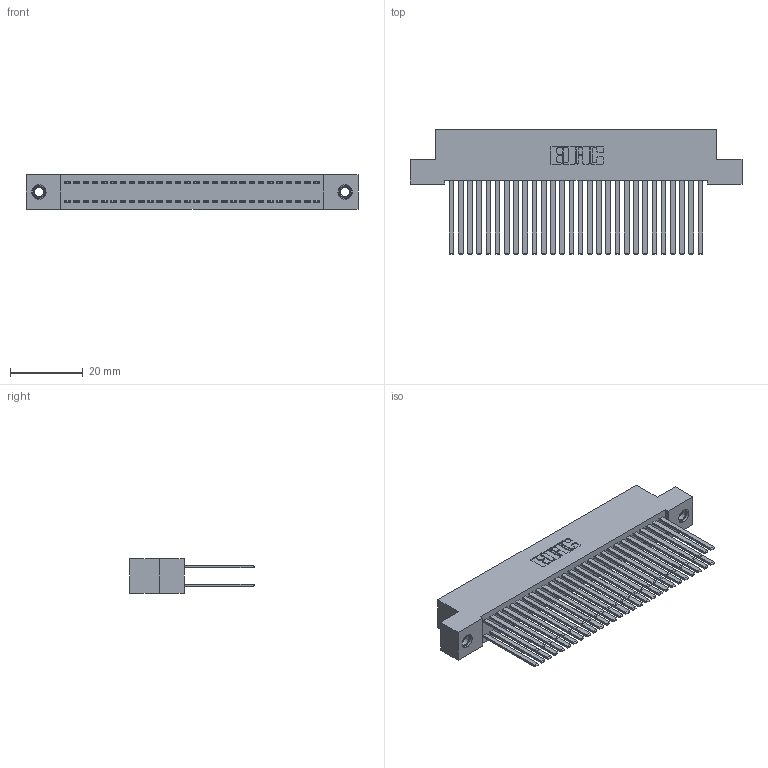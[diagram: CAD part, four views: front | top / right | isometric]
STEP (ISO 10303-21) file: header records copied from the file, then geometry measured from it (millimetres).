
FILE_DESCRIPTION (( 'STEP AP203' ), '1' );
FILE_NAME ('392-056-544-207.STEP', '2019-10-08T15:22:14', ( '' ), ( '' ), 'SwSTEP 2.0', 'SolidWorks 2016', '' );
FILE_SCHEMA (( 'CONFIG_CONTROL_DESIGN' ));
Length unit declared in the file: inch
Products named in the file (4): 342 Part_TI; 345-292-001_345-293-144; 345-250-001_345-250-005-103; 392-056-544-207
Assembly tree (59 placements, depth 2):
  392-056-544-207
    342 Part_TI
    345-292-001_345-293-144  x56
    345-250-001_345-250-005-103  x2
Bounding box: 91.44 x 34.3 x 9.4 mm (x, y, z)
Volume: 8921.9 mm3; surface area: 16377.5 mm2
Topology: 59 solids, 59 shells, 2746 faces, 8107 edges, 5322 vertices
Faces by surface type: plane 1890, cylinder 840, cone 12, torus 4
Entity records: 20694 total; most frequent: CARTESIAN_POINT 3425, ORIENTED_EDGE 3354, DIRECTION 2979, EDGE_CURVE 1677, VECTOR 1533, LINE 1533, VERTEX_POINT 1112, AXIS2_PLACEMENT_3D 723
